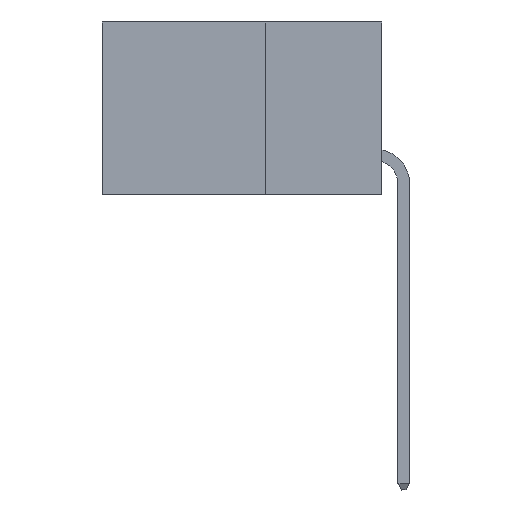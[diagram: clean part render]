
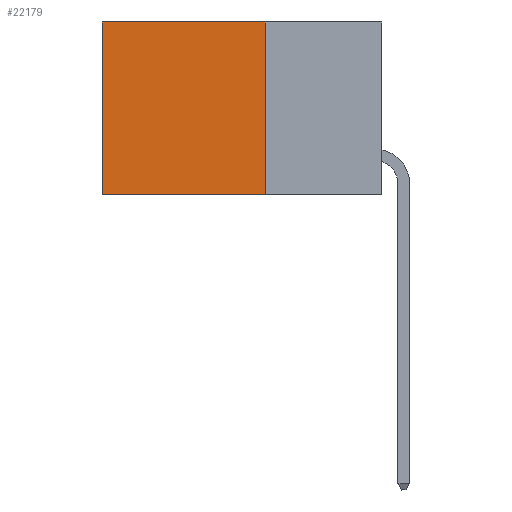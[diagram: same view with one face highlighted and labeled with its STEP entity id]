
A CAD part, left-side view. The second image highlights one B-rep face of the part: STEP entity #22179.
In plain terms, the highlighted planar face has unit normal (-1, 0, 0).
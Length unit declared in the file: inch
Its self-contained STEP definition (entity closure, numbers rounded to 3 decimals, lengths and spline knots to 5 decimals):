
#523 = ORIENTED_EDGE ( 'NONE', *, *, #37377, .T. ) ;
#1646 = VERTEX_POINT ( 'NONE', #32610 ) ;
#1893 = LINE ( 'NONE', #6997, #22610 ) ;
#2310 = LINE ( 'NONE', #8299, #38476 ) ;
#4734 = VECTOR ( 'NONE', #11520, 39.37008 ) ;
#5002 = CARTESIAN_POINT ( 'NONE',  ( 0.2875, 0.25, -0.37 ) ) ;
#5183 = CARTESIAN_POINT ( 'NONE',  ( 0.2875, 0.25, 0. ) ) ;
#6997 = CARTESIAN_POINT ( 'NONE',  ( 0.2875, 0.6, 0. ) ) ;
#7230 = EDGE_CURVE ( 'NONE', #17724, #1646, #2310, .T. ) ;
#7809 = CARTESIAN_POINT ( 'NONE',  ( 0.2875, 0.25, 0. ) ) ;
#8242 = CARTESIAN_POINT ( 'NONE',  ( 0.2875, 0.6, -0.37 ) ) ;
#8299 = CARTESIAN_POINT ( 'NONE',  ( 0.2875, 0.25, 0. ) ) ;
#11486 = ORIENTED_EDGE ( 'NONE', *, *, #35988, .F. ) ;
#11520 = DIRECTION ( 'NONE',  ( 0., 1., 0. ) ) ;
#11553 = EDGE_LOOP ( 'NONE', ( #523, #11486, #28445, #23452 ) ) ;
#13167 = EDGE_CURVE ( 'NONE', #17724, #31358, #28943, .T. ) ;
#17255 = DIRECTION ( 'NONE',  ( 0., 0., -1. ) ) ;
#17724 = VERTEX_POINT ( 'NONE', #5183 ) ;
#17818 = DIRECTION ( 'NONE',  ( 0., 1., 0. ) ) ;
#18194 = LINE ( 'NONE', #5002, #4734 ) ;
#22022 = VERTEX_POINT ( 'NONE', #8242 ) ;
#22179 = ADVANCED_FACE ( 'NONE', ( #23253 ), #28581, .F. ) ;
#22610 = VECTOR ( 'NONE', #40367, 39.37008 ) ;
#23253 = FACE_OUTER_BOUND ( 'NONE', #11553, .T. ) ;
#23452 = ORIENTED_EDGE ( 'NONE', *, *, #13167, .T. ) ;
#25581 = DIRECTION ( 'NONE',  ( 1., 0., 0. ) ) ;
#25943 = AXIS2_PLACEMENT_3D ( 'NONE', #35516, #25581, #38404 ) ;
#27915 = VECTOR ( 'NONE', #17818, 39.37008 ) ;
#28445 = ORIENTED_EDGE ( 'NONE', *, *, #7230, .F. ) ;
#28581 = PLANE ( 'NONE',  #25943 ) ;
#28943 = LINE ( 'NONE', #7809, #27915 ) ;
#31358 = VERTEX_POINT ( 'NONE', #38872 ) ;
#32610 = CARTESIAN_POINT ( 'NONE',  ( 0.2875, 0.25, -0.37 ) ) ;
#35516 = CARTESIAN_POINT ( 'NONE',  ( 0.2875, 0.25, 0. ) ) ;
#35988 = EDGE_CURVE ( 'NONE', #1646, #22022, #18194, .T. ) ;
#37377 = EDGE_CURVE ( 'NONE', #31358, #22022, #1893, .T. ) ;
#38404 = DIRECTION ( 'NONE',  ( 0., 0., -1. ) ) ;
#38476 = VECTOR ( 'NONE', #17255, 39.37008 ) ;
#38872 = CARTESIAN_POINT ( 'NONE',  ( 0.2875, 0.6, 0. ) ) ;
#40367 = DIRECTION ( 'NONE',  ( 0., 0., -1. ) ) ;
